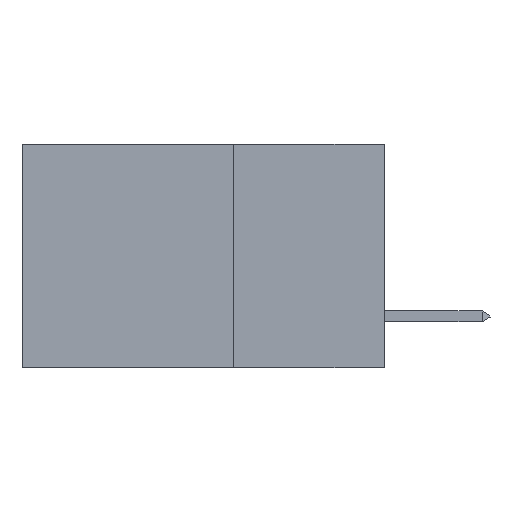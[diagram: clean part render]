
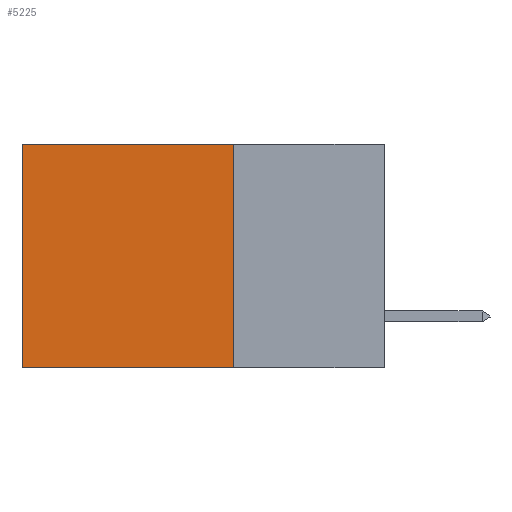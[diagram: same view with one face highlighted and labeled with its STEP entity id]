
A CAD part, left-side view. The second image highlights one B-rep face of the part: STEP entity #5225.
In plain terms, the highlighted planar face has unit normal (-1, 0, 0).
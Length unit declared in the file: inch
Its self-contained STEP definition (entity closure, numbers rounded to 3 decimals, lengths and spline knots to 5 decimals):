
#1940 = EDGE_LOOP ( 'NONE', ( #2355, #8713, #20397, #42573 ) ) ;
#2238 = CARTESIAN_POINT ( 'NONE',  ( 0.2875, 0.25, 0. ) ) ;
#2355 = ORIENTED_EDGE ( 'NONE', *, *, #4379, .T. ) ;
#3541 = FACE_OUTER_BOUND ( 'NONE', #1940, .T. ) ;
#4379 = EDGE_CURVE ( 'NONE', #12446, #40939, #44488, .T. ) ;
#5225 = ADVANCED_FACE ( 'NONE', ( #3541 ), #44613, .F. ) ;
#6881 = EDGE_CURVE ( 'NONE', #15019, #12446, #49493, .T. ) ;
#8713 = ORIENTED_EDGE ( 'NONE', *, *, #25577, .F. ) ;
#9209 = DIRECTION ( 'NONE',  ( 0., 0., -1. ) ) ;
#9266 = CARTESIAN_POINT ( 'NONE',  ( 0.2875, 0.25, -0.37 ) ) ;
#11126 = VECTOR ( 'NONE', #45183, 39.37008 ) ;
#12446 = VERTEX_POINT ( 'NONE', #16141 ) ;
#14052 = VECTOR ( 'NONE', #16667, 39.37008 ) ;
#14759 = CARTESIAN_POINT ( 'NONE',  ( 0.2875, 0.6, -0.37 ) ) ;
#15019 = VERTEX_POINT ( 'NONE', #25151 ) ;
#15916 = VECTOR ( 'NONE', #31551, 39.37008 ) ;
#16141 = CARTESIAN_POINT ( 'NONE',  ( 0.2875, 0.6, 0. ) ) ;
#16667 = DIRECTION ( 'NONE',  ( 0., 1., 0. ) ) ;
#20397 = ORIENTED_EDGE ( 'NONE', *, *, #24423, .F. ) ;
#24423 = EDGE_CURVE ( 'NONE', #15019, #46114, #39221, .T. ) ;
#24668 = VECTOR ( 'NONE', #9209, 39.37008 ) ;
#25151 = CARTESIAN_POINT ( 'NONE',  ( 0.2875, 0.25, 0. ) ) ;
#25577 = EDGE_CURVE ( 'NONE', #46114, #40939, #26037, .T. ) ;
#25738 = DIRECTION ( 'NONE',  ( 0., 0., -1. ) ) ;
#26037 = LINE ( 'NONE', #9266, #14052 ) ;
#27980 = CARTESIAN_POINT ( 'NONE',  ( 0.2875, 0.6, 0. ) ) ;
#28049 = CARTESIAN_POINT ( 'NONE',  ( 0.2875, 0.25, 0. ) ) ;
#31551 = DIRECTION ( 'NONE',  ( 0., 0., -1. ) ) ;
#33594 = CARTESIAN_POINT ( 'NONE',  ( 0.2875, 0.25, -0.37 ) ) ;
#33667 = AXIS2_PLACEMENT_3D ( 'NONE', #2238, #40589, #25738 ) ;
#39221 = LINE ( 'NONE', #28049, #15916 ) ;
#40589 = DIRECTION ( 'NONE',  ( 1., 0., 0. ) ) ;
#40829 = CARTESIAN_POINT ( 'NONE',  ( 0.2875, 0.25, 0. ) ) ;
#40939 = VERTEX_POINT ( 'NONE', #14759 ) ;
#42573 = ORIENTED_EDGE ( 'NONE', *, *, #6881, .T. ) ;
#44488 = LINE ( 'NONE', #27980, #24668 ) ;
#44613 = PLANE ( 'NONE',  #33667 ) ;
#45183 = DIRECTION ( 'NONE',  ( 0., 1., 0. ) ) ;
#46114 = VERTEX_POINT ( 'NONE', #33594 ) ;
#49493 = LINE ( 'NONE', #40829, #11126 ) ;
